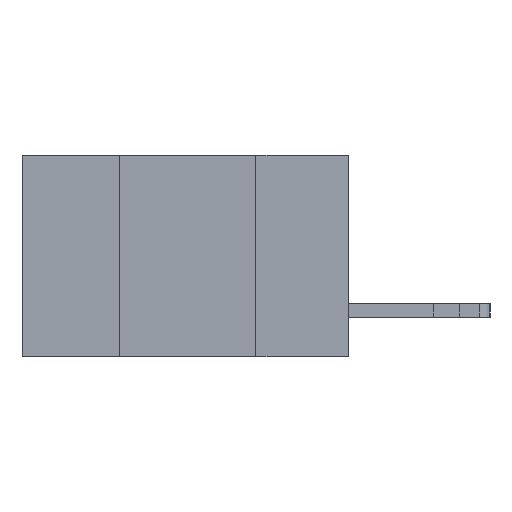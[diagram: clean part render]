
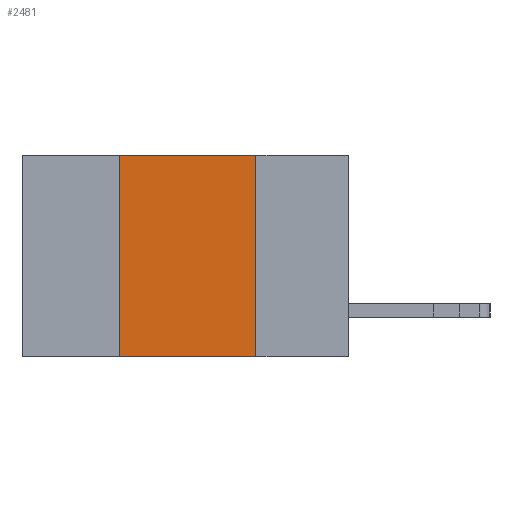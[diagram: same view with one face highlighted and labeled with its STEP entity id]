
A CAD part, left-side view. The second image highlights one B-rep face of the part: STEP entity #2481.
In plain terms, the highlighted planar face has unit normal (-1, 0, 0).
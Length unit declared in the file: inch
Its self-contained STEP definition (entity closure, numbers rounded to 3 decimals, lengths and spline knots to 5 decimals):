
#433 = VERTEX_POINT ( 'NONE', #16862 ) ;
#801 = DIRECTION ( 'NONE',  ( 0., 0., -1. ) ) ;
#837 = VECTOR ( 'NONE', #9544, 39.37008 ) ;
#972 = ORIENTED_EDGE ( 'NONE', *, *, #7178, .F. ) ;
#1006 = CARTESIAN_POINT ( 'NONE',  ( 0., 0.6, -0.37 ) ) ;
#1062 = DIRECTION ( 'NONE',  ( 0., -1., 0. ) ) ;
#2421 = LINE ( 'NONE', #1006, #12125 ) ;
#2481 = ADVANCED_FACE ( 'NONE', ( #12527 ), #7155, .F. ) ;
#2528 = CARTESIAN_POINT ( 'NONE',  ( 0., 0.42, 0. ) ) ;
#3935 = DIRECTION ( 'NONE',  ( 0., -1., 0. ) ) ;
#3973 = CARTESIAN_POINT ( 'NONE',  ( 0., 0.6, 0. ) ) ;
#4202 = VERTEX_POINT ( 'NONE', #2528 ) ;
#5094 = ORIENTED_EDGE ( 'NONE', *, *, #8447, .F. ) ;
#5098 = ORIENTED_EDGE ( 'NONE', *, *, #6594, .F. ) ;
#5380 = VECTOR ( 'NONE', #3935, 39.37008 ) ;
#5430 = VECTOR ( 'NONE', #8182, 39.37008 ) ;
#6285 = CARTESIAN_POINT ( 'NONE',  ( 0., 0.17, -0.37 ) ) ;
#6594 = EDGE_CURVE ( 'NONE', #433, #4202, #12303, .T. ) ;
#6624 = AXIS2_PLACEMENT_3D ( 'NONE', #13061, #12895, #801 ) ;
#7155 = PLANE ( 'NONE',  #6624 ) ;
#7178 = EDGE_CURVE ( 'NONE', #12211, #11102, #12726, .T. ) ;
#7664 = CARTESIAN_POINT ( 'NONE',  ( 0., 0.17, 0. ) ) ;
#8136 = EDGE_LOOP ( 'NONE', ( #972, #5094, #5098, #9448 ) ) ;
#8157 = CARTESIAN_POINT ( 'NONE',  ( 0., 0.17, -0.37 ) ) ;
#8182 = DIRECTION ( 'NONE',  ( 0., 0., -1. ) ) ;
#8447 = EDGE_CURVE ( 'NONE', #4202, #12211, #16118, .T. ) ;
#9151 = CARTESIAN_POINT ( 'NONE',  ( 0., 0.42, -0.37 ) ) ;
#9448 = ORIENTED_EDGE ( 'NONE', *, *, #16836, .T. ) ;
#9544 = DIRECTION ( 'NONE',  ( 0., 0., 1. ) ) ;
#11102 = VERTEX_POINT ( 'NONE', #6285 ) ;
#12125 = VECTOR ( 'NONE', #1062, 39.37008 ) ;
#12211 = VERTEX_POINT ( 'NONE', #7664 ) ;
#12303 = LINE ( 'NONE', #9151, #837 ) ;
#12527 = FACE_OUTER_BOUND ( 'NONE', #8136, .T. ) ;
#12726 = LINE ( 'NONE', #8157, #5430 ) ;
#12895 = DIRECTION ( 'NONE',  ( 1., 0., 0. ) ) ;
#13061 = CARTESIAN_POINT ( 'NONE',  ( 0., 0.6, 0. ) ) ;
#16118 = LINE ( 'NONE', #3973, #5380 ) ;
#16836 = EDGE_CURVE ( 'NONE', #433, #11102, #2421, .T. ) ;
#16862 = CARTESIAN_POINT ( 'NONE',  ( 0., 0.42, -0.37 ) ) ;
